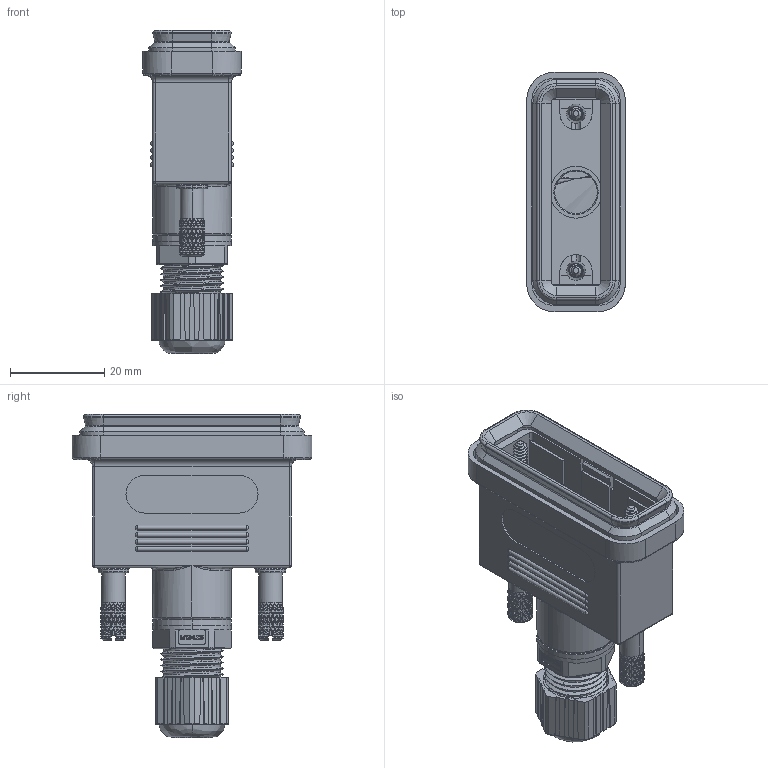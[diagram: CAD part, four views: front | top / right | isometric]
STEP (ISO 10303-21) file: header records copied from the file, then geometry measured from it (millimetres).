
FILE_DESCRIPTION (( 'STEP AP214' ), '1' );
FILE_NAME ('627-230-015-010.STEP', '2020-09-16T21:00:41', ( '' ), ( '' ), 'SwSTEP 2.0', 'SolidWorks 2020', '' );
FILE_SCHEMA (( 'AUTOMOTIVE_DESIGN' ));
Length unit declared in the file: millimetre
Products named in the file (9): Main Body 15; Clamp Nut; Cable Guide; Thumbscrew; Cable Seal; 627-230-015-010; Seal 15; O-Ring S; O-Ring L
Assembly tree (10 placements, depth 2):
  627-230-015-010
    Main Body 15
    O-Ring S  x2
    Thumbscrew  x2
    O-Ring L
    Cable Guide
    Cable Seal
    Clamp Nut
    Seal 15
Bounding box: 20.9 x 50.87 x 68.5 mm (x, y, z)
Volume: 6070 mm3; surface area: 19304.9 mm2
Topology: 9 solids, 10 shells, 2796 faces, 6451 edges, 3697 vertices
Faces by surface type: bspline 1567, cylinder 557, plane 545, cone 117, torus 10
Entity records: 89863 total; most frequent: CARTESIAN_POINT 54377, ORIENTED_EDGE 8842, DIRECTION 4513, EDGE_CURVE 4422, VERTEX_POINT 2623, B_SPLINE_CURVE_WITH_KNOTS 2321, EDGE_LOOP 1890, ADVANCED_FACE 1843
